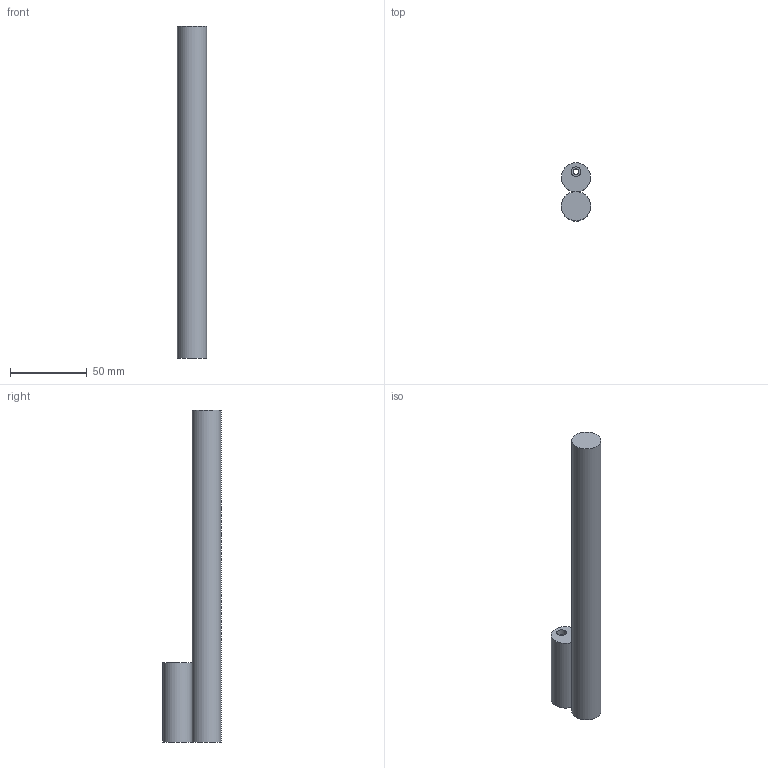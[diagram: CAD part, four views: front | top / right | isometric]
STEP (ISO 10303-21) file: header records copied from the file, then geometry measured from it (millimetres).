
FILE_DESCRIPTION(('FreeCAD Model'),'2;1');
FILE_NAME( 'AP9 simulated bolt.step', '2017-11-13T22:51:40',('Author'),(''), 'Open CASCADE STEP processor 6.8','FreeCAD','Unknown');
FILE_SCHEMA(('AUTOMOTIVE_DESIGN_CC2 { 1 2 10303 214 -1 1 5 4 }'));
Length unit declared in the file: millimetre
Products named in the file (1): Fusion
Bounding box: 19 x 38 x 216 mm (x, y, z)
Volume: 75252.4 mm3; surface area: 17688.2 mm2
Topology: 2 solids, 2 shells, 10 faces, 16 edges, 11 vertices
Faces by surface type: plane 5, cylinder 5
Full cylindrical faces by diameter (mm): 3.53 x1, 6.35 x1, 19 x1
Entity records: 504 total; most frequent: CARTESIAN_POINT 126, DIRECTION 70, ORIENTED_EDGE 32, PCURVE 32, DEFINITIONAL_REPRESENTATION 32, LINE 24, VECTOR 24, AXIS2_PLACEMENT_3D 22
